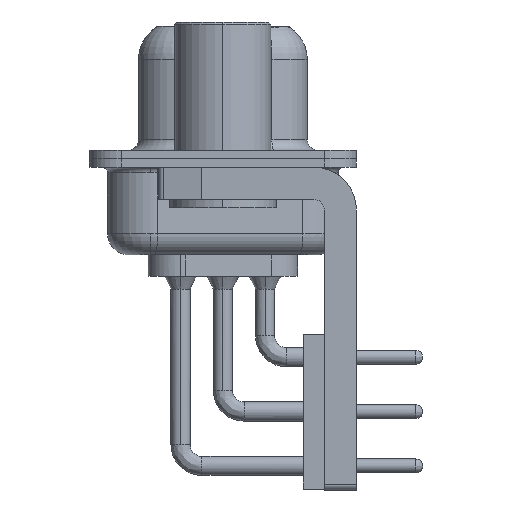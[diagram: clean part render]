
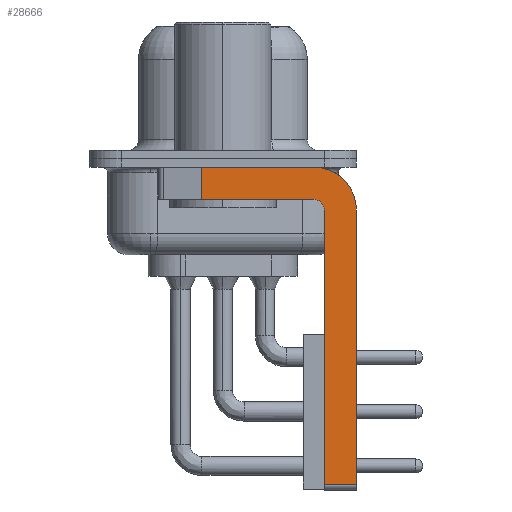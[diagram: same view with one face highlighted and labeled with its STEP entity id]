
A CAD part, left-side view. The second image highlights one B-rep face of the part: STEP entity #28666.
In plain terms, the highlighted planar face has unit normal (-1, 0, 0).
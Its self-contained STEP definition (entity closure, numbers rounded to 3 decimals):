
#570 = VERTEX_POINT ( 'NONE', #14980 ) ;
#718 = VERTEX_POINT ( 'NONE', #17449 ) ;
#792 = CARTESIAN_POINT ( 'NONE',  ( -2.9, -4.25, -2.4 ) ) ;
#1933 = VERTEX_POINT ( 'NONE', #22971 ) ;
#2545 = CARTESIAN_POINT ( 'NONE',  ( -2.9, 0.978, -1.9 ) ) ;
#3158 = AXIS2_PLACEMENT_3D ( 'NONE', #792, #20557, #3642 ) ;
#3642 = DIRECTION ( 'NONE',  ( 0., 0., -1. ) ) ;
#3689 = CARTESIAN_POINT ( 'NONE',  ( -2.9, -4.25, -2.4 ) ) ;
#3911 = VECTOR ( 'NONE', #25168, 1000. ) ;
#4678 = FACE_OUTER_BOUND ( 'NONE', #21032, .T. ) ;
#5746 = LINE ( 'NONE', #17074, #34821 ) ;
#6445 = ORIENTED_EDGE ( 'NONE', *, *, #30744, .F. ) ;
#6514 = DIRECTION ( 'NONE',  ( 0., 0., 1. ) ) ;
#7122 = CARTESIAN_POINT ( 'NONE',  ( -2.9, -6.25, -2.4 ) ) ;
#7463 = EDGE_CURVE ( 'NONE', #718, #15068, #13870, .T. ) ;
#8308 = VECTOR ( 'NONE', #11142, 1000. ) ;
#8997 = ORIENTED_EDGE ( 'NONE', *, *, #7463, .F. ) ;
#9168 = LINE ( 'NONE', #22376, #8308 ) ;
#10530 = VECTOR ( 'NONE', #21851, 1000. ) ;
#10892 = CARTESIAN_POINT ( 'NONE',  ( -2.9, -4.25, -1.9 ) ) ;
#11142 = DIRECTION ( 'NONE',  ( 0., 0., 1. ) ) ;
#11420 = LINE ( 'NONE', #7122, #10530 ) ;
#11686 = ORIENTED_EDGE ( 'NONE', *, *, #31345, .F. ) ;
#12743 = ORIENTED_EDGE ( 'NONE', *, *, #21202, .F. ) ;
#12901 = EDGE_CURVE ( 'NONE', #34043, #718, #9168, .T. ) ;
#13679 = PLANE ( 'NONE',  #35612 ) ;
#13870 = CIRCLE ( 'NONE', #24202, 0.5 ) ;
#14280 = CARTESIAN_POINT ( 'NONE',  ( -2.9, -4.75, -15.25 ) ) ;
#14980 = CARTESIAN_POINT ( 'NONE',  ( -2.9, 0.978, -0.4 ) ) ;
#15068 = VERTEX_POINT ( 'NONE', #17946 ) ;
#16505 = DIRECTION ( 'NONE',  ( 1., 0., 0. ) ) ;
#17074 = CARTESIAN_POINT ( 'NONE',  ( -2.9, -4.25, -15.25 ) ) ;
#17405 = VERTEX_POINT ( 'NONE', #23636 ) ;
#17449 = CARTESIAN_POINT ( 'NONE',  ( -2.9, -4.75, -2.4 ) ) ;
#17766 = CARTESIAN_POINT ( 'NONE',  ( -2.9, 3., -0.4 ) ) ;
#17946 = CARTESIAN_POINT ( 'NONE',  ( -2.9, -4.25, -1.9 ) ) ;
#18138 = ORIENTED_EDGE ( 'NONE', *, *, #21834, .T. ) ;
#20557 = DIRECTION ( 'NONE',  ( 1., 0., 0. ) ) ;
#20671 = EDGE_CURVE ( 'NONE', #34043, #17405, #5746, .T. ) ;
#21032 = EDGE_LOOP ( 'NONE', ( #6445, #18138, #12743, #8997, #32009, #30564, #32559, #11686 ) ) ;
#21202 = EDGE_CURVE ( 'NONE', #15068, #32022, #35666, .T. ) ;
#21834 = EDGE_CURVE ( 'NONE', #570, #32022, #27295, .T. ) ;
#21851 = DIRECTION ( 'NONE',  ( 0., 0., -1. ) ) ;
#22376 = CARTESIAN_POINT ( 'NONE',  ( -2.9, -4.75, -15.5 ) ) ;
#22708 = VECTOR ( 'NONE', #26276, 1000. ) ;
#22971 = CARTESIAN_POINT ( 'NONE',  ( -2.9, -4.25, -0.4 ) ) ;
#23467 = DIRECTION ( 'NONE',  ( -1., 0., 0. ) ) ;
#23574 = CIRCLE ( 'NONE', #3158, 2. ) ;
#23636 = CARTESIAN_POINT ( 'NONE',  ( -2.9, -6.25, -15.25 ) ) ;
#23638 = CARTESIAN_POINT ( 'NONE',  ( -2.9, 0.978, -1.9 ) ) ;
#24202 = AXIS2_PLACEMENT_3D ( 'NONE', #3689, #23467, #6514 ) ;
#24986 = DIRECTION ( 'NONE',  ( 0., 1., 0. ) ) ;
#25168 = DIRECTION ( 'NONE',  ( 0., 0., -1. ) ) ;
#26276 = DIRECTION ( 'NONE',  ( 0., -1., 0. ) ) ;
#27295 = LINE ( 'NONE', #2545, #3911 ) ;
#28666 = ADVANCED_FACE ( 'NONE', ( #4678 ), #13679, .F. ) ;
#29195 = CARTESIAN_POINT ( 'NONE',  ( -2.9, -6.25, -2.4 ) ) ;
#30164 = LINE ( 'NONE', #17766, #22708 ) ;
#30564 = ORIENTED_EDGE ( 'NONE', *, *, #20671, .T. ) ;
#30744 = EDGE_CURVE ( 'NONE', #570, #1933, #30164, .T. ) ;
#31345 = EDGE_CURVE ( 'NONE', #1933, #33628, #23574, .T. ) ;
#32009 = ORIENTED_EDGE ( 'NONE', *, *, #12901, .F. ) ;
#32022 = VERTEX_POINT ( 'NONE', #23638 ) ;
#32559 = ORIENTED_EDGE ( 'NONE', *, *, #35583, .F. ) ;
#33329 = CARTESIAN_POINT ( 'NONE',  ( -2.9, -4.25, -2.4 ) ) ;
#33628 = VERTEX_POINT ( 'NONE', #29195 ) ;
#33905 = DIRECTION ( 'NONE',  ( 0., -1., 0. ) ) ;
#34043 = VERTEX_POINT ( 'NONE', #14280 ) ;
#34789 = VECTOR ( 'NONE', #24986, 1000. ) ;
#34821 = VECTOR ( 'NONE', #33905, 1000. ) ;
#35583 = EDGE_CURVE ( 'NONE', #33628, #17405, #11420, .T. ) ;
#35612 = AXIS2_PLACEMENT_3D ( 'NONE', #33329, #16505, #36142 ) ;
#35666 = LINE ( 'NONE', #10892, #34789 ) ;
#36142 = DIRECTION ( 'NONE',  ( 0., 0., -1. ) ) ;
